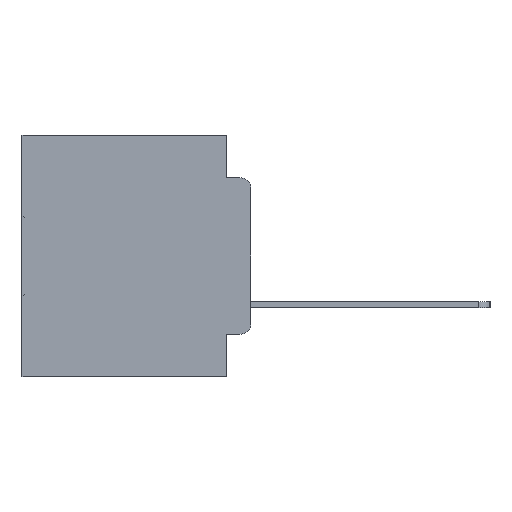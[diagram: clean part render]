
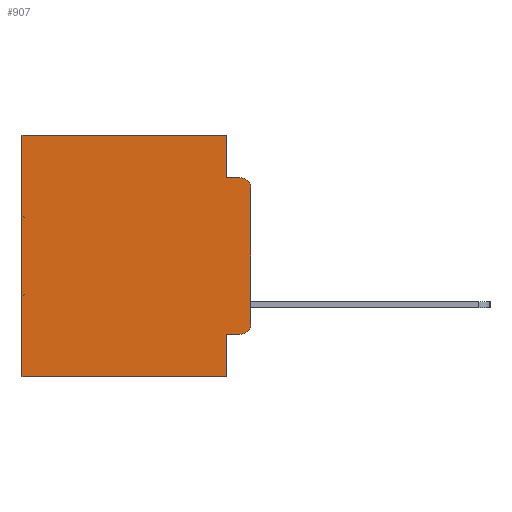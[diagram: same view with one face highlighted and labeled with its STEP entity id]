
A CAD part, left-side view. The second image highlights one B-rep face of the part: STEP entity #907.
In plain terms, the highlighted planar face has unit normal (-1, 0, 0).
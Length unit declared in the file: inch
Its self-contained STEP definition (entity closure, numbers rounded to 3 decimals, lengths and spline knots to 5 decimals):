
#13 = LINE ( 'NONE', #26701, #14597 ) ;
#406 = ORIENTED_EDGE ( 'NONE', *, *, #19661, .T. ) ;
#866 = ORIENTED_EDGE ( 'NONE', *, *, #22207, .F. ) ;
#907 = ADVANCED_FACE ( 'NONE', ( #9362 ), #23484, .F. ) ;
#1922 = ORIENTED_EDGE ( 'NONE', *, *, #18025, .F. ) ;
#2634 = ORIENTED_EDGE ( 'NONE', *, *, #10838, .T. ) ;
#2818 = ORIENTED_EDGE ( 'NONE', *, *, #8914, .T. ) ;
#3181 = DIRECTION ( 'NONE',  ( 0., 0., -1. ) ) ;
#3459 = DIRECTION ( 'NONE',  ( 0., 1., 0. ) ) ;
#3806 = VERTEX_POINT ( 'NONE', #12056 ) ;
#4827 = VECTOR ( 'NONE', #34010, 39.37008 ) ;
#4834 = DIRECTION ( 'NONE',  ( 0., 0., -1. ) ) ;
#4869 = VECTOR ( 'NONE', #19859, 39.37008 ) ;
#4890 = DIRECTION ( 'NONE',  ( 0., 0., -1. ) ) ;
#4935 = VERTEX_POINT ( 'NONE', #33695 ) ;
#5020 = DIRECTION ( 'NONE',  ( 1., 0., 0. ) ) ;
#5701 = CARTESIAN_POINT ( 'NONE',  ( 0.298, 0.473, 0. ) ) ;
#6096 = LINE ( 'NONE', #21193, #12823 ) ;
#6292 = EDGE_LOOP ( 'NONE', ( #25434, #25795, #27812, #29051, #23701, #406, #866, #1922, #2634, #2818 ) ) ;
#6336 = DIRECTION ( 'NONE',  ( -1., 0., 0. ) ) ;
#7418 = VERTEX_POINT ( 'NONE', #5701 ) ;
#8625 = VERTEX_POINT ( 'NONE', #26852 ) ;
#8914 = EDGE_CURVE ( 'NONE', #9057, #10770, #18537, .T. ) ;
#9057 = VERTEX_POINT ( 'NONE', #31097 ) ;
#9265 = CARTESIAN_POINT ( 'NONE',  ( 0.298, 0.051, -0.4115 ) ) ;
#9362 = FACE_OUTER_BOUND ( 'NONE', #6292, .T. ) ;
#10113 = EDGE_CURVE ( 'NONE', #8625, #10770, #23909, .T. ) ;
#10148 = AXIS2_PLACEMENT_3D ( 'NONE', #20476, #5020, #4834 ) ;
#10770 = VERTEX_POINT ( 'NONE', #11859 ) ;
#10838 = EDGE_CURVE ( 'NONE', #17877, #9057, #14282, .T. ) ;
#11683 = CARTESIAN_POINT ( 'NONE',  ( 0.298, 0.473, -0.5 ) ) ;
#11731 = DIRECTION ( 'NONE',  ( 0., 0., -1. ) ) ;
#11859 = CARTESIAN_POINT ( 'NONE',  ( 0.298, 0., -0.3915 ) ) ;
#12056 = CARTESIAN_POINT ( 'NONE',  ( 0.298, 0.051, -0.5 ) ) ;
#12823 = VECTOR ( 'NONE', #4890, 39.37008 ) ;
#13280 = DIRECTION ( 'NONE',  ( -1., 0., 0. ) ) ;
#14282 = LINE ( 'NONE', #9265, #4869 ) ;
#14597 = VECTOR ( 'NONE', #29074, 39.37008 ) ;
#14846 = CARTESIAN_POINT ( 'NONE',  ( 0.298, 0.051, -0.0885 ) ) ;
#15199 = EDGE_CURVE ( 'NONE', #4935, #7418, #19489, .T. ) ;
#15513 = VECTOR ( 'NONE', #22521, 39.37008 ) ;
#17055 = CARTESIAN_POINT ( 'NONE',  ( 0.298, 0., 0. ) ) ;
#17877 = VERTEX_POINT ( 'NONE', #30897 ) ;
#18025 = EDGE_CURVE ( 'NONE', #17877, #3806, #13, .T. ) ;
#18112 = VERTEX_POINT ( 'NONE', #11683 ) ;
#18510 = AXIS2_PLACEMENT_3D ( 'NONE', #22389, #6336, #24865 ) ;
#18537 = CIRCLE ( 'NONE', #30984, 0.02 ) ;
#18722 = CIRCLE ( 'NONE', #18510, 0.02 ) ;
#19489 = LINE ( 'NONE', #17055, #4827 ) ;
#19661 = EDGE_CURVE ( 'NONE', #7418, #18112, #6096, .T. ) ;
#19859 = DIRECTION ( 'NONE',  ( 0., -1., 0. ) ) ;
#20476 = CARTESIAN_POINT ( 'NONE',  ( 0.298, 0., 0. ) ) ;
#21193 = CARTESIAN_POINT ( 'NONE',  ( 0.298, 0.473, 0. ) ) ;
#21328 = EDGE_CURVE ( 'NONE', #4935, #26663, #32974, .T. ) ;
#22207 = EDGE_CURVE ( 'NONE', #3806, #18112, #29600, .T. ) ;
#22252 = LINE ( 'NONE', #14846, #15513 ) ;
#22389 = CARTESIAN_POINT ( 'NONE',  ( 0.298, 0.02, -0.1085 ) ) ;
#22453 = CARTESIAN_POINT ( 'NONE',  ( 0.298, 0., -0.5 ) ) ;
#22521 = DIRECTION ( 'NONE',  ( 0., -1., 0. ) ) ;
#23009 = CARTESIAN_POINT ( 'NONE',  ( 0.298, 0.02, -0.0885 ) ) ;
#23248 = VECTOR ( 'NONE', #3459, 39.37008 ) ;
#23484 = PLANE ( 'NONE',  #10148 ) ;
#23701 = ORIENTED_EDGE ( 'NONE', *, *, #15199, .T. ) ;
#23909 = LINE ( 'NONE', #29572, #29493 ) ;
#24865 = DIRECTION ( 'NONE',  ( 0., 0., -1. ) ) ;
#25434 = ORIENTED_EDGE ( 'NONE', *, *, #10113, .F. ) ;
#25795 = ORIENTED_EDGE ( 'NONE', *, *, #31075, .T. ) ;
#26663 = VERTEX_POINT ( 'NONE', #26904 ) ;
#26701 = CARTESIAN_POINT ( 'NONE',  ( 0.298, 0.051, 0. ) ) ;
#26852 = CARTESIAN_POINT ( 'NONE',  ( 0.298, 0., -0.1085 ) ) ;
#26904 = CARTESIAN_POINT ( 'NONE',  ( 0.298, 0.051, -0.0885 ) ) ;
#27309 = VERTEX_POINT ( 'NONE', #23009 ) ;
#27812 = ORIENTED_EDGE ( 'NONE', *, *, #27879, .F. ) ;
#27879 = EDGE_CURVE ( 'NONE', #26663, #27309, #22252, .T. ) ;
#28288 = CARTESIAN_POINT ( 'NONE',  ( 0.298, 0.02, -0.3915 ) ) ;
#29051 = ORIENTED_EDGE ( 'NONE', *, *, #21328, .F. ) ;
#29074 = DIRECTION ( 'NONE',  ( 0., 0., -1. ) ) ;
#29493 = VECTOR ( 'NONE', #3181, 39.37008 ) ;
#29572 = CARTESIAN_POINT ( 'NONE',  ( 0.298, 0., 0. ) ) ;
#29600 = LINE ( 'NONE', #22453, #23248 ) ;
#30699 = DIRECTION ( 'NONE',  ( 0., 0., -1. ) ) ;
#30897 = CARTESIAN_POINT ( 'NONE',  ( 0.298, 0.051, -0.4115 ) ) ;
#30984 = AXIS2_PLACEMENT_3D ( 'NONE', #28288, #13280, #30699 ) ;
#31075 = EDGE_CURVE ( 'NONE', #8625, #27309, #18722, .T. ) ;
#31097 = CARTESIAN_POINT ( 'NONE',  ( 0.298, 0.02, -0.4115 ) ) ;
#31725 = CARTESIAN_POINT ( 'NONE',  ( 0.298, 0.051, 0. ) ) ;
#32246 = VECTOR ( 'NONE', #11731, 39.37008 ) ;
#32974 = LINE ( 'NONE', #31725, #32246 ) ;
#33695 = CARTESIAN_POINT ( 'NONE',  ( 0.298, 0.051, 0. ) ) ;
#34010 = DIRECTION ( 'NONE',  ( 0., 1., 0. ) ) ;
